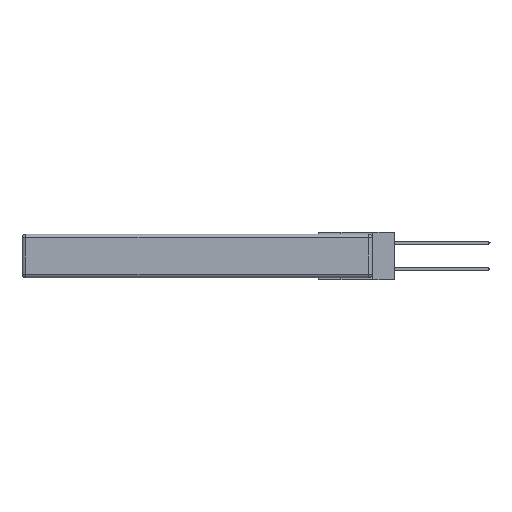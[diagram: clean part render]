
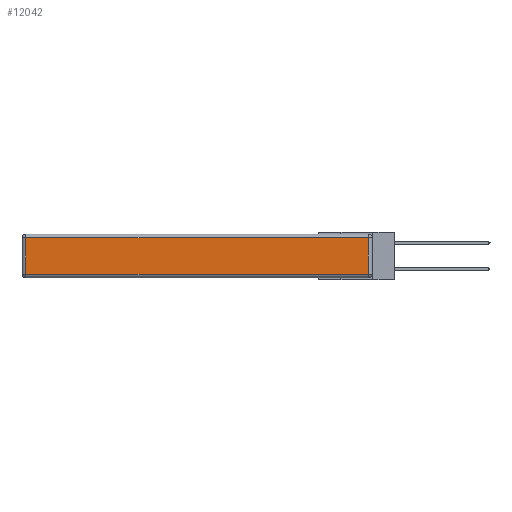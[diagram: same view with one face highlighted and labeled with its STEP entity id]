
A CAD part, left-side view. The second image highlights one B-rep face of the part: STEP entity #12042.
In plain terms, the highlighted planar face has unit normal (-1, 0, 0).
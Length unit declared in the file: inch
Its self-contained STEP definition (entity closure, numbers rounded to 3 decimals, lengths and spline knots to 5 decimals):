
#90 = LINE ( 'NONE', #4686, #3744 ) ;
#440 = ORIENTED_EDGE ( 'NONE', *, *, #6066, .T. ) ;
#707 = VECTOR ( 'NONE', #11952, 39.37008 ) ;
#1368 = EDGE_CURVE ( 'NONE', #4868, #1617, #11552, .T. ) ;
#1482 = CARTESIAN_POINT ( 'NONE',  ( 0., 2.72, -0.313 ) ) ;
#1617 = VERTEX_POINT ( 'NONE', #1482 ) ;
#2672 = EDGE_CURVE ( 'NONE', #5119, #4868, #4607, .T. ) ;
#3028 = CARTESIAN_POINT ( 'NONE',  ( 0., 2.72, -0.343 ) ) ;
#3744 = VECTOR ( 'NONE', #9586, 39.37008 ) ;
#3800 = CARTESIAN_POINT ( 'NONE',  ( 0., 0., -0.343 ) ) ;
#4607 = LINE ( 'NONE', #8383, #9862 ) ;
#4686 = CARTESIAN_POINT ( 'NONE',  ( 0., 0.03, -0.343 ) ) ;
#4868 = VERTEX_POINT ( 'NONE', #6474 ) ;
#5119 = VERTEX_POINT ( 'NONE', #8950 ) ;
#5262 = ORIENTED_EDGE ( 'NONE', *, *, #7742, .T. ) ;
#5405 = ORIENTED_EDGE ( 'NONE', *, *, #2672, .T. ) ;
#5474 = VECTOR ( 'NONE', #6587, 39.37008 ) ;
#5637 = PLANE ( 'NONE',  #6840 ) ;
#5859 = CARTESIAN_POINT ( 'NONE',  ( 0., 0.03, -0.313 ) ) ;
#6066 = EDGE_CURVE ( 'NONE', #1617, #10398, #8905, .T. ) ;
#6474 = CARTESIAN_POINT ( 'NONE',  ( 0., 2.72, -0.03 ) ) ;
#6549 = DIRECTION ( 'NONE',  ( 0., 0., 1. ) ) ;
#6587 = DIRECTION ( 'NONE',  ( 0., 0., -1. ) ) ;
#6840 = AXIS2_PLACEMENT_3D ( 'NONE', #3800, #10251, #6549 ) ;
#6943 = FACE_OUTER_BOUND ( 'NONE', #8761, .T. ) ;
#7548 = ORIENTED_EDGE ( 'NONE', *, *, #1368, .T. ) ;
#7742 = EDGE_CURVE ( 'NONE', #10398, #5119, #90, .T. ) ;
#8383 = CARTESIAN_POINT ( 'NONE',  ( 0., 2.75, -0.03 ) ) ;
#8761 = EDGE_LOOP ( 'NONE', ( #440, #5262, #5405, #7548 ) ) ;
#8905 = LINE ( 'NONE', #10261, #707 ) ;
#8950 = CARTESIAN_POINT ( 'NONE',  ( 0., 0.03, -0.03 ) ) ;
#9282 = DIRECTION ( 'NONE',  ( 0., 1., 0. ) ) ;
#9586 = DIRECTION ( 'NONE',  ( 0., 0., 1. ) ) ;
#9862 = VECTOR ( 'NONE', #9282, 39.37008 ) ;
#10251 = DIRECTION ( 'NONE',  ( -1., 0., 0. ) ) ;
#10261 = CARTESIAN_POINT ( 'NONE',  ( 0., 0., -0.313 ) ) ;
#10398 = VERTEX_POINT ( 'NONE', #5859 ) ;
#11552 = LINE ( 'NONE', #3028, #5474 ) ;
#11952 = DIRECTION ( 'NONE',  ( 0., -1., 0. ) ) ;
#12042 = ADVANCED_FACE ( 'NONE', ( #6943 ), #5637, .T. ) ;
